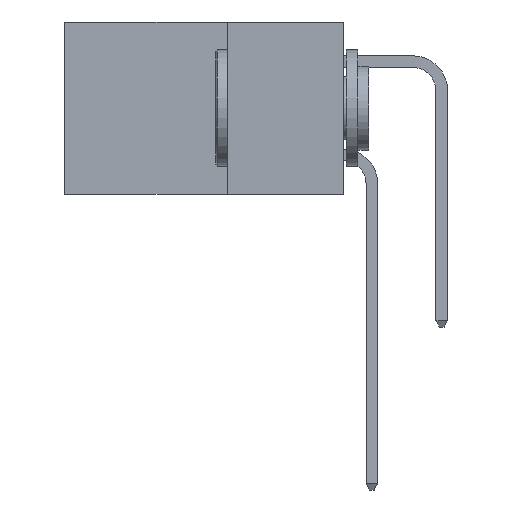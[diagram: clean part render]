
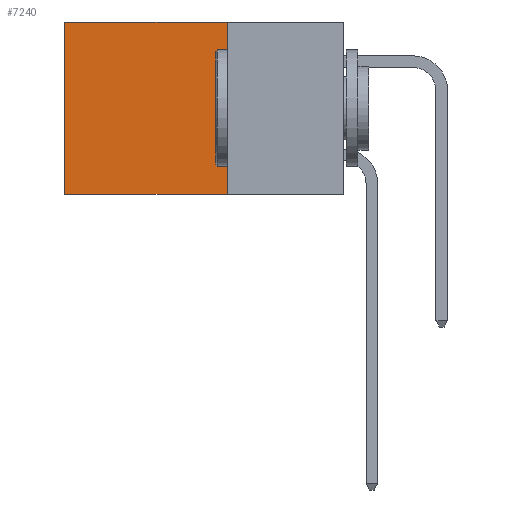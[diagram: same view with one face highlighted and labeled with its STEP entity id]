
A CAD part, left-side view. The second image highlights one B-rep face of the part: STEP entity #7240.
In plain terms, the highlighted planar face has unit normal (-1, 0, 0).
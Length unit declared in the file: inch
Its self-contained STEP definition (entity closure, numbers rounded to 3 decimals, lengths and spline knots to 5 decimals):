
#195 = CARTESIAN_POINT ( 'NONE',  ( 0.2615, 0.6, -0.37 ) ) ;
#389 = LINE ( 'NONE', #11789, #10282 ) ;
#700 = DIRECTION ( 'NONE',  ( 0., 1., 0. ) ) ;
#2098 = DIRECTION ( 'NONE',  ( 0., 0., -1. ) ) ;
#3830 = CARTESIAN_POINT ( 'NONE',  ( 0.2615, 0.6, 0. ) ) ;
#5056 = LINE ( 'NONE', #15217, #14264 ) ;
#5345 = VERTEX_POINT ( 'NONE', #3830 ) ;
#5560 = EDGE_CURVE ( 'NONE', #19668, #5345, #389, .T. ) ;
#6231 = CARTESIAN_POINT ( 'NONE',  ( 0.2615, 0.25, -0.37 ) ) ;
#7240 = ADVANCED_FACE ( 'NONE', ( #23340 ), #19052, .F. ) ;
#7263 = CARTESIAN_POINT ( 'NONE',  ( 0.2615, 0.25, -0.37 ) ) ;
#7459 = CARTESIAN_POINT ( 'NONE',  ( 0.2615, 0.6, -0.37 ) ) ;
#7595 = VECTOR ( 'NONE', #2098, 39.37008 ) ;
#8175 = LINE ( 'NONE', #195, #7595 ) ;
#9905 = DIRECTION ( 'NONE',  ( 0., 0., -1. ) ) ;
#10282 = VECTOR ( 'NONE', #700, 39.37008 ) ;
#11726 = EDGE_CURVE ( 'NONE', #5345, #17919, #8175, .T. ) ;
#11789 = CARTESIAN_POINT ( 'NONE',  ( 0.2615, 0.25, 0. ) ) ;
#11974 = VECTOR ( 'NONE', #12011, 39.37008 ) ;
#12011 = DIRECTION ( 'NONE',  ( 0., 1., 0. ) ) ;
#12127 = AXIS2_PLACEMENT_3D ( 'NONE', #6231, #20869, #9905 ) ;
#13886 = EDGE_LOOP ( 'NONE', ( #18544, #22135, #22271, #15784 ) ) ;
#14264 = VECTOR ( 'NONE', #17069, 39.37008 ) ;
#15217 = CARTESIAN_POINT ( 'NONE',  ( 0.2615, 0.25, -0.37 ) ) ;
#15671 = CARTESIAN_POINT ( 'NONE',  ( 0.2615, 0.25, 0. ) ) ;
#15784 = ORIENTED_EDGE ( 'NONE', *, *, #5560, .T. ) ;
#16322 = LINE ( 'NONE', #19352, #11974 ) ;
#16689 = EDGE_CURVE ( 'NONE', #19668, #19105, #5056, .T. ) ;
#17069 = DIRECTION ( 'NONE',  ( 0., 0., -1. ) ) ;
#17919 = VERTEX_POINT ( 'NONE', #7459 ) ;
#18544 = ORIENTED_EDGE ( 'NONE', *, *, #11726, .T. ) ;
#19052 = PLANE ( 'NONE',  #12127 ) ;
#19105 = VERTEX_POINT ( 'NONE', #7263 ) ;
#19352 = CARTESIAN_POINT ( 'NONE',  ( 0.2615, 0.25, -0.37 ) ) ;
#19668 = VERTEX_POINT ( 'NONE', #15671 ) ;
#19674 = EDGE_CURVE ( 'NONE', #19105, #17919, #16322, .T. ) ;
#20869 = DIRECTION ( 'NONE',  ( 1., 0., 0. ) ) ;
#22135 = ORIENTED_EDGE ( 'NONE', *, *, #19674, .F. ) ;
#22271 = ORIENTED_EDGE ( 'NONE', *, *, #16689, .F. ) ;
#23340 = FACE_OUTER_BOUND ( 'NONE', #13886, .T. ) ;
